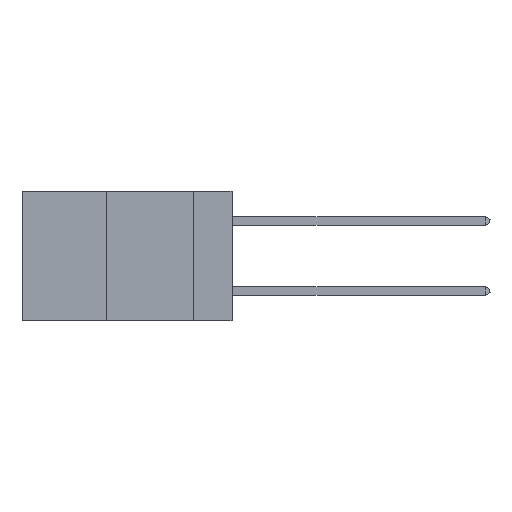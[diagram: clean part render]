
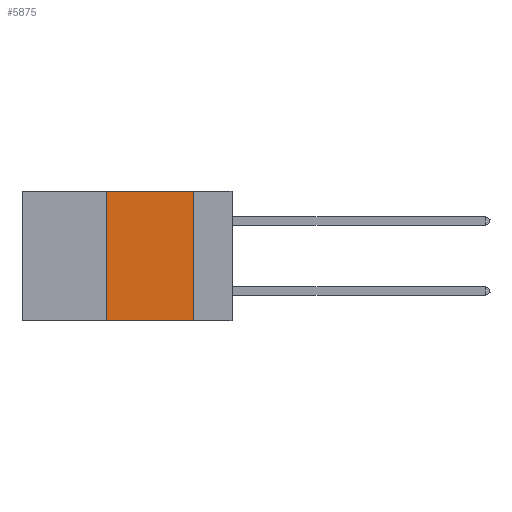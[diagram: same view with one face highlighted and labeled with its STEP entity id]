
A CAD part, left-side view. The second image highlights one B-rep face of the part: STEP entity #5875.
In plain terms, the highlighted planar face has unit normal (-1, 0, 0).
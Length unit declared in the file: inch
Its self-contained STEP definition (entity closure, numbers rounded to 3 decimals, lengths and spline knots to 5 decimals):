
#476 = VERTEX_POINT ( 'NONE', #31182 ) ;
#967 = LINE ( 'NONE', #19980, #13734 ) ;
#1669 = EDGE_CURVE ( 'NONE', #4673, #9856, #11128, .T. ) ;
#2627 = CARTESIAN_POINT ( 'NONE',  ( 0., 0.36, 0. ) ) ;
#3292 = FACE_OUTER_BOUND ( 'NONE', #31105, .T. ) ;
#3902 = PLANE ( 'NONE',  #6909 ) ;
#4673 = VERTEX_POINT ( 'NONE', #30209 ) ;
#4821 = DIRECTION ( 'NONE',  ( 0., 0., -1. ) ) ;
#5760 = CARTESIAN_POINT ( 'NONE',  ( 0., 0.11, -0.37 ) ) ;
#5875 = ADVANCED_FACE ( 'NONE', ( #3292 ), #3902, .F. ) ;
#6495 = DIRECTION ( 'NONE',  ( 1., 0., 0. ) ) ;
#6909 = AXIS2_PLACEMENT_3D ( 'NONE', #14144, #6495, #24779 ) ;
#7246 = EDGE_CURVE ( 'NONE', #476, #9856, #21570, .T. ) ;
#9495 = VECTOR ( 'NONE', #28511, 39.37008 ) ;
#9614 = ORIENTED_EDGE ( 'NONE', *, *, #10340, .F. ) ;
#9856 = VERTEX_POINT ( 'NONE', #5760 ) ;
#10340 = EDGE_CURVE ( 'NONE', #4673, #12830, #19056, .T. ) ;
#10569 = CARTESIAN_POINT ( 'NONE',  ( 0., 0.6, -0.37 ) ) ;
#11128 = LINE ( 'NONE', #10569, #24732 ) ;
#12830 = VERTEX_POINT ( 'NONE', #2627 ) ;
#13734 = VECTOR ( 'NONE', #17507, 39.37008 ) ;
#14144 = CARTESIAN_POINT ( 'NONE',  ( 0., 0.6, 0. ) ) ;
#15956 = VECTOR ( 'NONE', #4821, 39.37008 ) ;
#17507 = DIRECTION ( 'NONE',  ( 0., -1., 0. ) ) ;
#17523 = CARTESIAN_POINT ( 'NONE',  ( 0., 0.11, 0. ) ) ;
#19056 = LINE ( 'NONE', #22344, #9495 ) ;
#19980 = CARTESIAN_POINT ( 'NONE',  ( 0., 0.6, 0. ) ) ;
#21570 = LINE ( 'NONE', #17523, #15956 ) ;
#22344 = CARTESIAN_POINT ( 'NONE',  ( 0., 0.36, 0. ) ) ;
#22789 = EDGE_CURVE ( 'NONE', #12830, #476, #967, .T. ) ;
#24732 = VECTOR ( 'NONE', #28735, 39.37008 ) ;
#24779 = DIRECTION ( 'NONE',  ( 0., 0., -1. ) ) ;
#28324 = ORIENTED_EDGE ( 'NONE', *, *, #1669, .T. ) ;
#28511 = DIRECTION ( 'NONE',  ( 0., 0., 1. ) ) ;
#28735 = DIRECTION ( 'NONE',  ( 0., -1., 0. ) ) ;
#28767 = ORIENTED_EDGE ( 'NONE', *, *, #7246, .F. ) ;
#28888 = ORIENTED_EDGE ( 'NONE', *, *, #22789, .F. ) ;
#30209 = CARTESIAN_POINT ( 'NONE',  ( 0., 0.36, -0.37 ) ) ;
#31105 = EDGE_LOOP ( 'NONE', ( #28767, #28888, #9614, #28324 ) ) ;
#31182 = CARTESIAN_POINT ( 'NONE',  ( 0., 0.11, 0. ) ) ;
